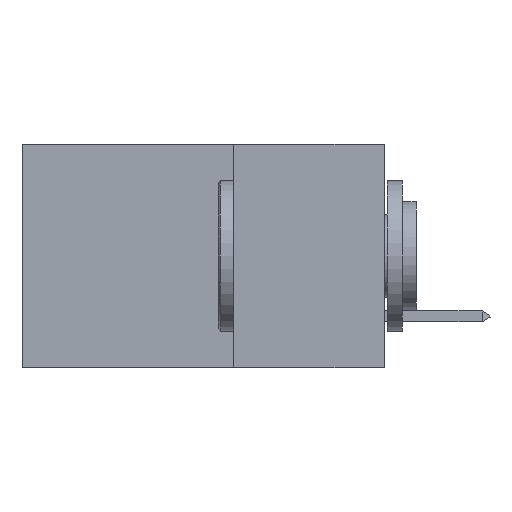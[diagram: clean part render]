
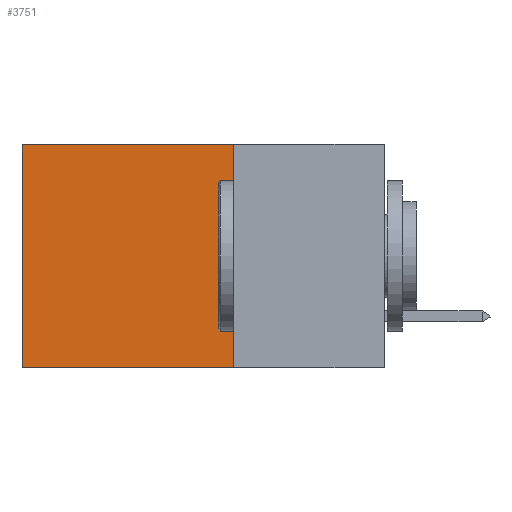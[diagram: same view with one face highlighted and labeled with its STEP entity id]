
A CAD part, left-side view. The second image highlights one B-rep face of the part: STEP entity #3751.
In plain terms, the highlighted planar face has unit normal (-1, 0, 0).
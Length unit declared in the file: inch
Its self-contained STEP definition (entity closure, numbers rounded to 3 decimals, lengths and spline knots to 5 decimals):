
#72 = VERTEX_POINT ( 'NONE', #1870 ) ;
#460 = DIRECTION ( 'NONE',  ( 0., 0., -1. ) ) ;
#594 = CARTESIAN_POINT ( 'NONE',  ( 0.2875, 0.6, 0. ) ) ;
#1538 = AXIS2_PLACEMENT_3D ( 'NONE', #3526, #4533, #11737 ) ;
#1616 = EDGE_CURVE ( 'NONE', #4361, #3302, #2129, .T. ) ;
#1870 = CARTESIAN_POINT ( 'NONE',  ( 0.2875, 0.6, 0. ) ) ;
#2055 = DIRECTION ( 'NONE',  ( 0., 1., 0. ) ) ;
#2088 = CARTESIAN_POINT ( 'NONE',  ( 0.2875, 0.25, -0.37 ) ) ;
#2129 = LINE ( 'NONE', #2088, #12987 ) ;
#2130 = CARTESIAN_POINT ( 'NONE',  ( 0.2875, 0.25, 0. ) ) ;
#2941 = VECTOR ( 'NONE', #7119, 39.37008 ) ;
#3302 = VERTEX_POINT ( 'NONE', #6170 ) ;
#3313 = EDGE_LOOP ( 'NONE', ( #6374, #9785, #11674, #12868 ) ) ;
#3322 = EDGE_CURVE ( 'NONE', #11272, #4361, #4365, .T. ) ;
#3526 = CARTESIAN_POINT ( 'NONE',  ( 0.2875, 0.25, 0. ) ) ;
#3751 = ADVANCED_FACE ( 'NONE', ( #6501 ), #9673, .F. ) ;
#3966 = EDGE_CURVE ( 'NONE', #72, #3302, #7140, .T. ) ;
#4044 = CARTESIAN_POINT ( 'NONE',  ( 0.2875, 0.25, -0.37 ) ) ;
#4361 = VERTEX_POINT ( 'NONE', #4044 ) ;
#4365 = LINE ( 'NONE', #2130, #2941 ) ;
#4533 = DIRECTION ( 'NONE',  ( 1., 0., 0. ) ) ;
#6170 = CARTESIAN_POINT ( 'NONE',  ( 0.2875, 0.6, -0.37 ) ) ;
#6374 = ORIENTED_EDGE ( 'NONE', *, *, #3966, .T. ) ;
#6501 = FACE_OUTER_BOUND ( 'NONE', #3313, .T. ) ;
#6702 = CARTESIAN_POINT ( 'NONE',  ( 0.2875, 0.25, 0. ) ) ;
#7119 = DIRECTION ( 'NONE',  ( 0., 0., -1. ) ) ;
#7140 = LINE ( 'NONE', #594, #7442 ) ;
#7442 = VECTOR ( 'NONE', #460, 39.37008 ) ;
#8271 = CARTESIAN_POINT ( 'NONE',  ( 0.2875, 0.25, 0. ) ) ;
#8714 = DIRECTION ( 'NONE',  ( 0., 1., 0. ) ) ;
#8892 = EDGE_CURVE ( 'NONE', #11272, #72, #12563, .T. ) ;
#9555 = VECTOR ( 'NONE', #8714, 39.37008 ) ;
#9673 = PLANE ( 'NONE',  #1538 ) ;
#9785 = ORIENTED_EDGE ( 'NONE', *, *, #1616, .F. ) ;
#11272 = VERTEX_POINT ( 'NONE', #8271 ) ;
#11674 = ORIENTED_EDGE ( 'NONE', *, *, #3322, .F. ) ;
#11737 = DIRECTION ( 'NONE',  ( 0., 0., -1. ) ) ;
#12563 = LINE ( 'NONE', #6702, #9555 ) ;
#12868 = ORIENTED_EDGE ( 'NONE', *, *, #8892, .T. ) ;
#12987 = VECTOR ( 'NONE', #2055, 39.37008 ) ;
